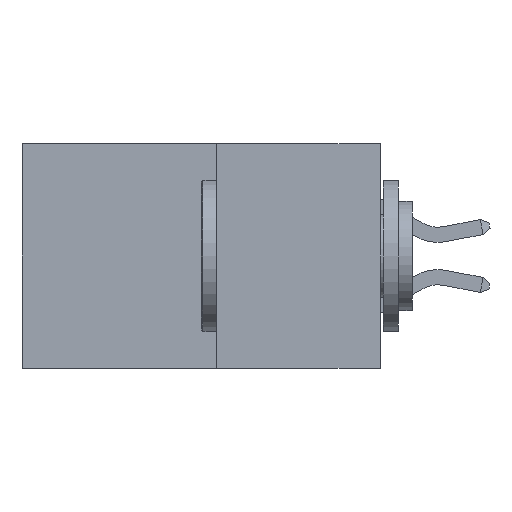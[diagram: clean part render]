
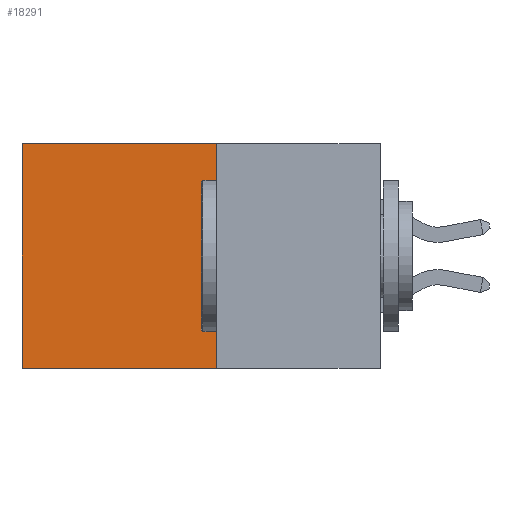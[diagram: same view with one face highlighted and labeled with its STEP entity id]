
A CAD part, left-side view. The second image highlights one B-rep face of the part: STEP entity #18291.
In plain terms, the highlighted planar face has unit normal (-1, 0, 0).
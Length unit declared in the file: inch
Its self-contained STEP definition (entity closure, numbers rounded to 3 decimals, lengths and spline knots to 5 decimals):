
#4 = VERTEX_POINT ( 'NONE', #12131 ) ;
#1029 = LINE ( 'NONE', #7688, #12420 ) ;
#1240 = CARTESIAN_POINT ( 'NONE',  ( 0.277, 0.27, -0.37 ) ) ;
#1959 = VERTEX_POINT ( 'NONE', #16519 ) ;
#1995 = EDGE_CURVE ( 'NONE', #1959, #4, #16266, .T. ) ;
#2764 = DIRECTION ( 'NONE',  ( 0., 0., -1. ) ) ;
#2828 = DIRECTION ( 'NONE',  ( 0., 1., 0. ) ) ;
#3859 = DIRECTION ( 'NONE',  ( 0., 0., -1. ) ) ;
#3865 = CARTESIAN_POINT ( 'NONE',  ( 0.277, 0.59, -0.37 ) ) ;
#3916 = VECTOR ( 'NONE', #16559, 39.37008 ) ;
#6263 = CARTESIAN_POINT ( 'NONE',  ( 0.277, 0.27, 0. ) ) ;
#6412 = VERTEX_POINT ( 'NONE', #11972 ) ;
#6487 = VECTOR ( 'NONE', #2828, 39.37008 ) ;
#7688 = CARTESIAN_POINT ( 'NONE',  ( 0.277, 0.27, -0.37 ) ) ;
#7707 = ORIENTED_EDGE ( 'NONE', *, *, #10199, .T. ) ;
#7785 = DIRECTION ( 'NONE',  ( 0., 0., -1. ) ) ;
#7918 = EDGE_LOOP ( 'NONE', ( #7707, #14943, #9509, #15841 ) ) ;
#9509 = ORIENTED_EDGE ( 'NONE', *, *, #10005, .F. ) ;
#9540 = CARTESIAN_POINT ( 'NONE',  ( 0.277, 0.27, -0.37 ) ) ;
#9977 = AXIS2_PLACEMENT_3D ( 'NONE', #10408, #12000, #2764 ) ;
#10005 = EDGE_CURVE ( 'NONE', #1959, #19901, #1029, .T. ) ;
#10199 = EDGE_CURVE ( 'NONE', #4, #6412, #17738, .T. ) ;
#10408 = CARTESIAN_POINT ( 'NONE',  ( 0.277, 0.27, -0.37 ) ) ;
#11972 = CARTESIAN_POINT ( 'NONE',  ( 0.277, 0.59, -0.37 ) ) ;
#12000 = DIRECTION ( 'NONE',  ( 1., 0., 0. ) ) ;
#12131 = CARTESIAN_POINT ( 'NONE',  ( 0.277, 0.59, 0. ) ) ;
#12420 = VECTOR ( 'NONE', #7785, 39.37008 ) ;
#14893 = EDGE_CURVE ( 'NONE', #19901, #6412, #18821, .T. ) ;
#14943 = ORIENTED_EDGE ( 'NONE', *, *, #14893, .F. ) ;
#15841 = ORIENTED_EDGE ( 'NONE', *, *, #1995, .T. ) ;
#16266 = LINE ( 'NONE', #6263, #3916 ) ;
#16519 = CARTESIAN_POINT ( 'NONE',  ( 0.277, 0.27, 0. ) ) ;
#16559 = DIRECTION ( 'NONE',  ( 0., 1., 0. ) ) ;
#16724 = FACE_OUTER_BOUND ( 'NONE', #7918, .T. ) ;
#17260 = VECTOR ( 'NONE', #3859, 39.37008 ) ;
#17738 = LINE ( 'NONE', #3865, #17260 ) ;
#18291 = ADVANCED_FACE ( 'NONE', ( #16724 ), #19718, .F. ) ;
#18821 = LINE ( 'NONE', #1240, #6487 ) ;
#19718 = PLANE ( 'NONE',  #9977 ) ;
#19901 = VERTEX_POINT ( 'NONE', #9540 ) ;
